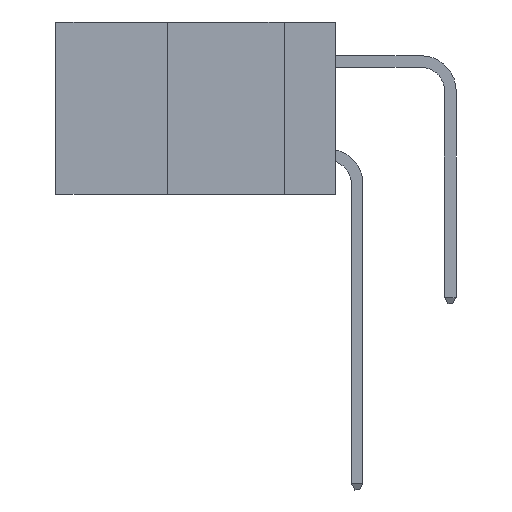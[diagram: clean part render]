
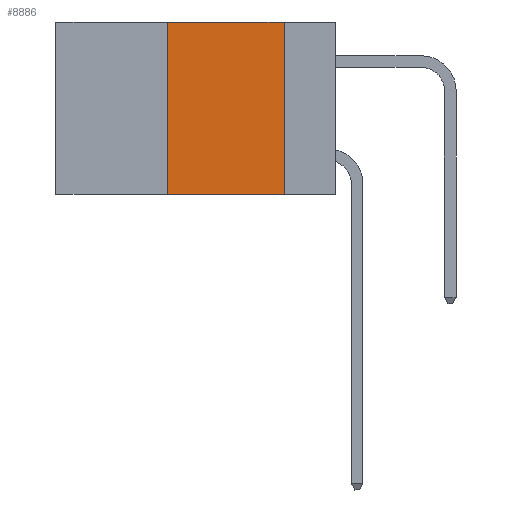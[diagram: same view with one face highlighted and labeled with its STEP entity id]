
A CAD part, left-side view. The second image highlights one B-rep face of the part: STEP entity #8886.
In plain terms, the highlighted planar face has unit normal (-1, 0, 0).
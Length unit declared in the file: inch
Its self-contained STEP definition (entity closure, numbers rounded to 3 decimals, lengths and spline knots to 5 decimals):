
#197 = CARTESIAN_POINT ( 'NONE',  ( 0., 0.11, 0. ) ) ;
#682 = CARTESIAN_POINT ( 'NONE',  ( 0., 0.11, 0. ) ) ;
#1348 = VECTOR ( 'NONE', #11173, 39.37008 ) ;
#1869 = EDGE_LOOP ( 'NONE', ( #6981, #2347, #2930, #5396 ) ) ;
#2166 = VECTOR ( 'NONE', #5415, 39.37008 ) ;
#2347 = ORIENTED_EDGE ( 'NONE', *, *, #10291, .F. ) ;
#2691 = DIRECTION ( 'NONE',  ( 1., 0., 0. ) ) ;
#2930 = ORIENTED_EDGE ( 'NONE', *, *, #5227, .F. ) ;
#3583 = VECTOR ( 'NONE', #7230, 39.37008 ) ;
#3725 = VERTEX_POINT ( 'NONE', #197 ) ;
#4037 = EDGE_CURVE ( 'NONE', #3725, #5045, #8231, .T. ) ;
#5045 = VERTEX_POINT ( 'NONE', #9788 ) ;
#5095 = VERTEX_POINT ( 'NONE', #8031 ) ;
#5175 = FACE_OUTER_BOUND ( 'NONE', #1869, .T. ) ;
#5227 = EDGE_CURVE ( 'NONE', #8057, #5095, #7148, .T. ) ;
#5396 = ORIENTED_EDGE ( 'NONE', *, *, #7090, .T. ) ;
#5415 = DIRECTION ( 'NONE',  ( 0., -1., 0. ) ) ;
#5462 = CARTESIAN_POINT ( 'NONE',  ( 0., 0.36, 0. ) ) ;
#6365 = PLANE ( 'NONE',  #9596 ) ;
#6981 = ORIENTED_EDGE ( 'NONE', *, *, #4037, .F. ) ;
#7030 = CARTESIAN_POINT ( 'NONE',  ( 0., 0.36, -0.37 ) ) ;
#7090 = EDGE_CURVE ( 'NONE', #8057, #5045, #11827, .T. ) ;
#7148 = LINE ( 'NONE', #5462, #11602 ) ;
#7230 = DIRECTION ( 'NONE',  ( 0., 0., -1. ) ) ;
#8031 = CARTESIAN_POINT ( 'NONE',  ( 0., 0.36, 0. ) ) ;
#8057 = VERTEX_POINT ( 'NONE', #7030 ) ;
#8231 = LINE ( 'NONE', #682, #3583 ) ;
#8777 = LINE ( 'NONE', #10331, #1348 ) ;
#8886 = ADVANCED_FACE ( 'NONE', ( #5175 ), #6365, .F. ) ;
#9152 = DIRECTION ( 'NONE',  ( 0., 0., 1. ) ) ;
#9163 = DIRECTION ( 'NONE',  ( 0., 0., -1. ) ) ;
#9596 = AXIS2_PLACEMENT_3D ( 'NONE', #10020, #2691, #9163 ) ;
#9788 = CARTESIAN_POINT ( 'NONE',  ( 0., 0.11, -0.37 ) ) ;
#10020 = CARTESIAN_POINT ( 'NONE',  ( 0., 0.6, 0. ) ) ;
#10291 = EDGE_CURVE ( 'NONE', #5095, #3725, #8777, .T. ) ;
#10331 = CARTESIAN_POINT ( 'NONE',  ( 0., 0.6, 0. ) ) ;
#10855 = CARTESIAN_POINT ( 'NONE',  ( 0., 0.6, -0.37 ) ) ;
#11173 = DIRECTION ( 'NONE',  ( 0., -1., 0. ) ) ;
#11602 = VECTOR ( 'NONE', #9152, 39.37008 ) ;
#11827 = LINE ( 'NONE', #10855, #2166 ) ;
